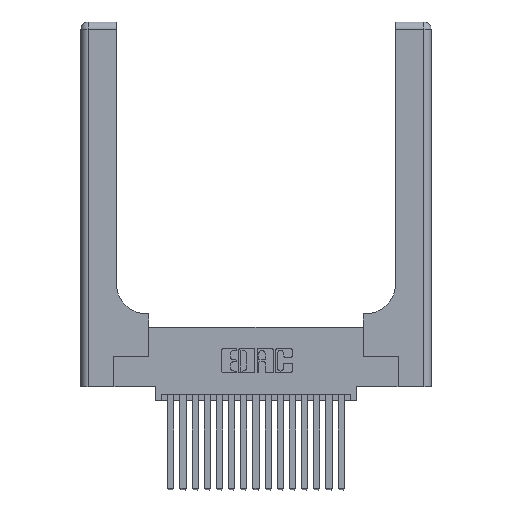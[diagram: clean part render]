
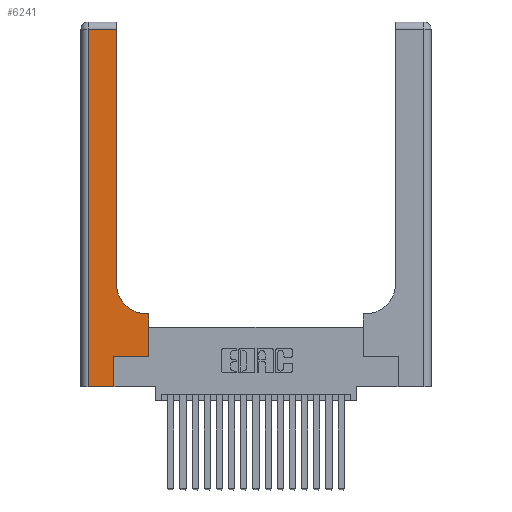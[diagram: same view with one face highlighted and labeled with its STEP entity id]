
A CAD part, top view. The second image highlights one B-rep face of the part: STEP entity #6241.
In plain terms, the highlighted planar face has unit normal (0, 0, 1).
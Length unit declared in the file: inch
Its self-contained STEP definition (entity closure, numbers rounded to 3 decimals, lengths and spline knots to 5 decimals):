
#461 = LINE ( 'NONE', #4295, #8629 ) ;
#468 = CARTESIAN_POINT ( 'NONE',  ( 0.269, 0., 0.37 ) ) ;
#868 = CARTESIAN_POINT ( 'NONE',  ( 0.5585, 0.6, 0.37 ) ) ;
#1320 = CARTESIAN_POINT ( 'NONE',  ( 0.5585, 0.25, 0.37 ) ) ;
#1762 = VERTEX_POINT ( 'NONE', #1320 ) ;
#2411 = CARTESIAN_POINT ( 'NONE',  ( 0., 2.94, 0.37 ) ) ;
#2443 = ORIENTED_EDGE ( 'NONE', *, *, #6732, .T. ) ;
#2558 = CIRCLE ( 'NONE', #6303, 0.25 ) ;
#2885 = VERTEX_POINT ( 'NONE', #5136 ) ;
#3136 = CARTESIAN_POINT ( 'NONE',  ( 0.269, 0., 0.37 ) ) ;
#3395 = CARTESIAN_POINT ( 'NONE',  ( 0.2915, 0.85, 0.37 ) ) ;
#3527 = LINE ( 'NONE', #9757, #19815 ) ;
#4030 = VECTOR ( 'NONE', #16846, 39.37008 ) ;
#4295 = CARTESIAN_POINT ( 'NONE',  ( 0.269, 0.25, 0.37 ) ) ;
#4345 = CARTESIAN_POINT ( 'NONE',  ( 0.2915, 2.94, 0.37 ) ) ;
#4413 = EDGE_CURVE ( 'NONE', #9514, #15545, #14268, .T. ) ;
#4781 = EDGE_CURVE ( 'NONE', #2885, #9514, #3527, .T. ) ;
#4948 = DIRECTION ( 'NONE',  ( -1., 0., 0. ) ) ;
#5136 = CARTESIAN_POINT ( 'NONE',  ( 0.06, 0., 0.37 ) ) ;
#5166 = EDGE_LOOP ( 'NONE', ( #7416, #13412, #20534, #13664, #12176, #12765, #13954, #2443, #14271 ) ) ;
#5708 = DIRECTION ( 'NONE',  ( -1., 0., 0. ) ) ;
#5850 = DIRECTION ( 'NONE',  ( 0., 0., -1. ) ) ;
#5874 = VECTOR ( 'NONE', #12767, 39.37008 ) ;
#6026 = CARTESIAN_POINT ( 'NONE',  ( 0.06, 2.94, 0.37 ) ) ;
#6122 = VERTEX_POINT ( 'NONE', #3395 ) ;
#6241 = ADVANCED_FACE ( 'NONE', ( #19223 ), #17851, .F. ) ;
#6303 = AXIS2_PLACEMENT_3D ( 'NONE', #15281, #5850, #16830 ) ;
#6496 = VECTOR ( 'NONE', #9212, 39.37008 ) ;
#6544 = EDGE_CURVE ( 'NONE', #1762, #13513, #10264, .T. ) ;
#6732 = EDGE_CURVE ( 'NONE', #13513, #16894, #7255, .T. ) ;
#6756 = CARTESIAN_POINT ( 'NONE',  ( 0.2915, 3., 0.37 ) ) ;
#6991 = DIRECTION ( 'NONE',  ( -1., 0., 0. ) ) ;
#7255 = LINE ( 'NONE', #11337, #15124 ) ;
#7416 = ORIENTED_EDGE ( 'NONE', *, *, #18761, .T. ) ;
#8629 = VECTOR ( 'NONE', #10722, 39.37008 ) ;
#8879 = LINE ( 'NONE', #19889, #4030 ) ;
#9212 = DIRECTION ( 'NONE',  ( 0., 1., 0. ) ) ;
#9514 = VERTEX_POINT ( 'NONE', #468 ) ;
#9757 = CARTESIAN_POINT ( 'NONE',  ( 0., 0., 0.37 ) ) ;
#10126 = CARTESIAN_POINT ( 'NONE',  ( 0., 3., 0.37 ) ) ;
#10264 = LINE ( 'NONE', #15469, #6496 ) ;
#10722 = DIRECTION ( 'NONE',  ( 1., 0., 0. ) ) ;
#11337 = CARTESIAN_POINT ( 'NONE',  ( 0.2915, 0.6, 0.37 ) ) ;
#11419 = VECTOR ( 'NONE', #19328, 39.37008 ) ;
#12176 = ORIENTED_EDGE ( 'NONE', *, *, #4413, .T. ) ;
#12451 = VECTOR ( 'NONE', #5708, 39.37008 ) ;
#12765 = ORIENTED_EDGE ( 'NONE', *, *, #17362, .T. ) ;
#12767 = DIRECTION ( 'NONE',  ( 0., 1., 0. ) ) ;
#12868 = CARTESIAN_POINT ( 'NONE',  ( 0.5415, 0.6, 0.37 ) ) ;
#12928 = DIRECTION ( 'NONE',  ( 1., 0., 0. ) ) ;
#13412 = ORIENTED_EDGE ( 'NONE', *, *, #14735, .T. ) ;
#13429 = AXIS2_PLACEMENT_3D ( 'NONE', #10126, #16368, #6991 ) ;
#13513 = VERTEX_POINT ( 'NONE', #868 ) ;
#13608 = VERTEX_POINT ( 'NONE', #6026 ) ;
#13664 = ORIENTED_EDGE ( 'NONE', *, *, #4781, .T. ) ;
#13954 = ORIENTED_EDGE ( 'NONE', *, *, #6544, .T. ) ;
#14268 = LINE ( 'NONE', #3136, #5874 ) ;
#14271 = ORIENTED_EDGE ( 'NONE', *, *, #19925, .T. ) ;
#14735 = EDGE_CURVE ( 'NONE', #17915, #13608, #16543, .T. ) ;
#15124 = VECTOR ( 'NONE', #4948, 39.37008 ) ;
#15281 = CARTESIAN_POINT ( 'NONE',  ( 0.5415, 0.85, 0.37 ) ) ;
#15469 = CARTESIAN_POINT ( 'NONE',  ( 0.5585, 0.25, 0.37 ) ) ;
#15535 = LINE ( 'NONE', #6756, #11419 ) ;
#15545 = VERTEX_POINT ( 'NONE', #17407 ) ;
#16368 = DIRECTION ( 'NONE',  ( 0., 0., -1. ) ) ;
#16543 = LINE ( 'NONE', #2411, #12451 ) ;
#16830 = DIRECTION ( 'NONE',  ( 1., 0., 0. ) ) ;
#16846 = DIRECTION ( 'NONE',  ( 0., -1., 0. ) ) ;
#16894 = VERTEX_POINT ( 'NONE', #12868 ) ;
#17362 = EDGE_CURVE ( 'NONE', #15545, #1762, #461, .T. ) ;
#17407 = CARTESIAN_POINT ( 'NONE',  ( 0.269, 0.25, 0.37 ) ) ;
#17851 = PLANE ( 'NONE',  #13429 ) ;
#17915 = VERTEX_POINT ( 'NONE', #4345 ) ;
#18344 = EDGE_CURVE ( 'NONE', #13608, #2885, #8879, .T. ) ;
#18761 = EDGE_CURVE ( 'NONE', #6122, #17915, #15535, .T. ) ;
#19223 = FACE_OUTER_BOUND ( 'NONE', #5166, .T. ) ;
#19328 = DIRECTION ( 'NONE',  ( 0., 1., 0. ) ) ;
#19815 = VECTOR ( 'NONE', #12928, 39.37008 ) ;
#19889 = CARTESIAN_POINT ( 'NONE',  ( 0.06, 3., 0.37 ) ) ;
#19925 = EDGE_CURVE ( 'NONE', #16894, #6122, #2558, .T. ) ;
#20534 = ORIENTED_EDGE ( 'NONE', *, *, #18344, .T. ) ;
